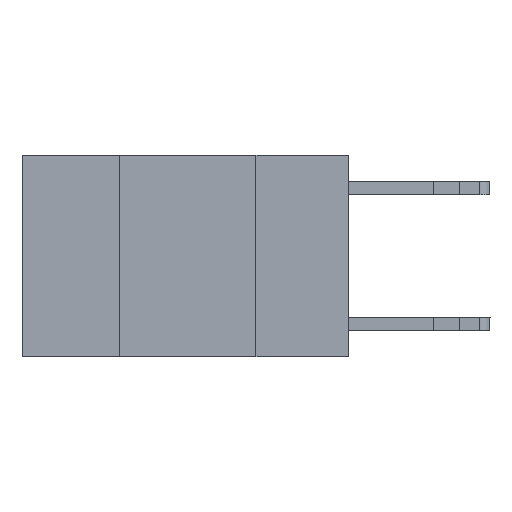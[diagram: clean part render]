
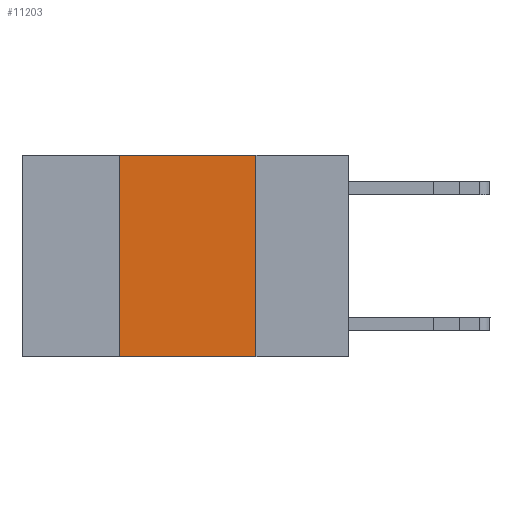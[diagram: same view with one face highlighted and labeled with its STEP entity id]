
A CAD part, left-side view. The second image highlights one B-rep face of the part: STEP entity #11203.
In plain terms, the highlighted planar face has unit normal (-1, 0, 0).
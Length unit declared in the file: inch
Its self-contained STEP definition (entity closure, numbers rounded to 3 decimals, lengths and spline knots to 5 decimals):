
#144 = PLANE ( 'NONE',  #3202 ) ;
#236 = EDGE_CURVE ( 'NONE', #13560, #6527, #1713, .T. ) ;
#1128 = VECTOR ( 'NONE', #12523, 39.37008 ) ;
#1368 = DIRECTION ( 'NONE',  ( 1., 0., 0. ) ) ;
#1713 = LINE ( 'NONE', #9604, #4894 ) ;
#2246 = DIRECTION ( 'NONE',  ( 0., 0., 1. ) ) ;
#2433 = DIRECTION ( 'NONE',  ( 0., -1., 0. ) ) ;
#2508 = FACE_OUTER_BOUND ( 'NONE', #15354, .T. ) ;
#3202 = AXIS2_PLACEMENT_3D ( 'NONE', #13459, #1368, #9848 ) ;
#3316 = LINE ( 'NONE', #9682, #6904 ) ;
#3376 = EDGE_CURVE ( 'NONE', #10356, #5434, #3896, .T. ) ;
#3710 = ORIENTED_EDGE ( 'NONE', *, *, #4089, .T. ) ;
#3896 = LINE ( 'NONE', #15550, #13610 ) ;
#4089 = EDGE_CURVE ( 'NONE', #10356, #6527, #3316, .T. ) ;
#4894 = VECTOR ( 'NONE', #7163, 39.37008 ) ;
#5380 = CARTESIAN_POINT ( 'NONE',  ( 0., 0.17, -0.37 ) ) ;
#5434 = VERTEX_POINT ( 'NONE', #13220 ) ;
#6187 = ORIENTED_EDGE ( 'NONE', *, *, #7735, .F. ) ;
#6527 = VERTEX_POINT ( 'NONE', #5380 ) ;
#6719 = CARTESIAN_POINT ( 'NONE',  ( 0., 0.17, 0. ) ) ;
#6904 = VECTOR ( 'NONE', #2433, 39.37008 ) ;
#7031 = CARTESIAN_POINT ( 'NONE',  ( 0., 0.42, -0.37 ) ) ;
#7163 = DIRECTION ( 'NONE',  ( 0., 0., -1. ) ) ;
#7546 = LINE ( 'NONE', #11334, #1128 ) ;
#7735 = EDGE_CURVE ( 'NONE', #5434, #13560, #7546, .T. ) ;
#8258 = ORIENTED_EDGE ( 'NONE', *, *, #236, .F. ) ;
#9604 = CARTESIAN_POINT ( 'NONE',  ( 0., 0.17, 0. ) ) ;
#9682 = CARTESIAN_POINT ( 'NONE',  ( 0., 0.6, -0.37 ) ) ;
#9848 = DIRECTION ( 'NONE',  ( 0., 0., -1. ) ) ;
#10356 = VERTEX_POINT ( 'NONE', #7031 ) ;
#11203 = ADVANCED_FACE ( 'NONE', ( #2508 ), #144, .F. ) ;
#11334 = CARTESIAN_POINT ( 'NONE',  ( 0., 0.6, 0. ) ) ;
#12523 = DIRECTION ( 'NONE',  ( 0., -1., 0. ) ) ;
#12650 = ORIENTED_EDGE ( 'NONE', *, *, #3376, .F. ) ;
#13220 = CARTESIAN_POINT ( 'NONE',  ( 0., 0.42, 0. ) ) ;
#13459 = CARTESIAN_POINT ( 'NONE',  ( 0., 0.6, 0. ) ) ;
#13560 = VERTEX_POINT ( 'NONE', #6719 ) ;
#13610 = VECTOR ( 'NONE', #2246, 39.37008 ) ;
#15354 = EDGE_LOOP ( 'NONE', ( #8258, #6187, #12650, #3710 ) ) ;
#15550 = CARTESIAN_POINT ( 'NONE',  ( 0., 0.42, 0. ) ) ;
